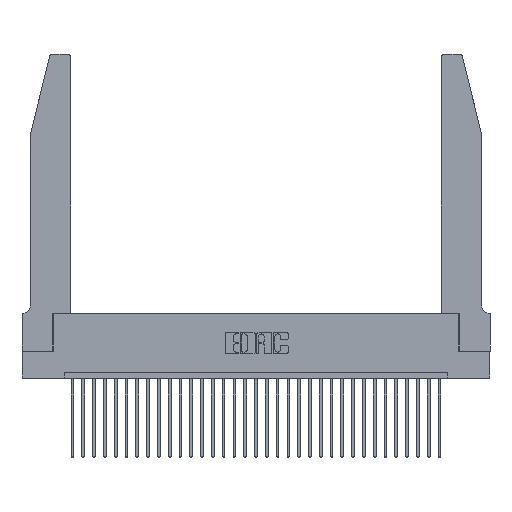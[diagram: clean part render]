
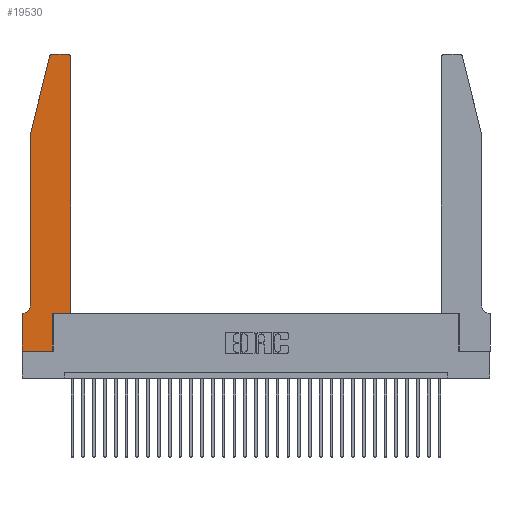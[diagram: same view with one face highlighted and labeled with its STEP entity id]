
A CAD part, top view. The second image highlights one B-rep face of the part: STEP entity #19530.
In plain terms, the highlighted planar face has unit normal (0, 0, 1).
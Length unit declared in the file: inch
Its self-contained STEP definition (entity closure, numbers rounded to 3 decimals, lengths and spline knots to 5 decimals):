
#37 = LINE ( 'NONE', #31479, #9733 ) ;
#382 = CARTESIAN_POINT ( 'NONE',  ( 0.0055, 0.35, 0.37 ) ) ;
#477 = ORIENTED_EDGE ( 'NONE', *, *, #24067, .T. ) ;
#713 = VERTEX_POINT ( 'NONE', #25484 ) ;
#748 = LINE ( 'NONE', #21684, #1137 ) ;
#1137 = VECTOR ( 'NONE', #14346, 39.37008 ) ;
#1479 = EDGE_LOOP ( 'NONE', ( #14843, #12441, #16678, #8493, #11657, #11386, #14791, #8676, #29667, #477, #28879, #24973 ) ) ;
#1513 = CARTESIAN_POINT ( 'NONE',  ( 0.284, 2.75, 0.37 ) ) ;
#1635 = CARTESIAN_POINT ( 'NONE',  ( 0.4505, 0.35, 0.37 ) ) ;
#1834 = AXIS2_PLACEMENT_3D ( 'NONE', #31867, #12397, #14784 ) ;
#1895 = VECTOR ( 'NONE', #10445, 39.37008 ) ;
#2207 = DIRECTION ( 'NONE',  ( 0., 1., 0. ) ) ;
#2646 = LINE ( 'NONE', #12282, #1895 ) ;
#2649 = CARTESIAN_POINT ( 'NONE',  ( 0.4505, 2.72, 0.37 ) ) ;
#2924 = DIRECTION ( 'NONE',  ( 0., 0., -1. ) ) ;
#3272 = VERTEX_POINT ( 'NONE', #19927 ) ;
#3446 = CARTESIAN_POINT ( 'NONE',  ( 0.0755, 0.42, 0.37 ) ) ;
#3865 = VERTEX_POINT ( 'NONE', #7511 ) ;
#4053 = CARTESIAN_POINT ( 'NONE',  ( 0.4505, 0.35, 0.37 ) ) ;
#4207 = DIRECTION ( 'NONE',  ( 0., 1., 0. ) ) ;
#4376 = EDGE_CURVE ( 'NONE', #12136, #10088, #5441, .T. ) ;
#4532 = DIRECTION ( 'NONE',  ( 1., 0., 0. ) ) ;
#4702 = CIRCLE ( 'NONE', #26055, 0.03 ) ;
#5030 = DIRECTION ( 'NONE',  ( -1., 0., 0. ) ) ;
#5145 = EDGE_CURVE ( 'NONE', #3272, #30229, #15882, .T. ) ;
#5441 = LINE ( 'NONE', #31015, #24458 ) ;
#7511 = CARTESIAN_POINT ( 'NONE',  ( 0., 0.35, 0.37 ) ) ;
#7933 = EDGE_CURVE ( 'NONE', #28340, #26289, #18375, .T. ) ;
#8493 = ORIENTED_EDGE ( 'NONE', *, *, #7933, .T. ) ;
#8676 = ORIENTED_EDGE ( 'NONE', *, *, #4376, .T. ) ;
#9013 = CARTESIAN_POINT ( 'NONE',  ( 0.2865, 0.35, 0.37 ) ) ;
#9733 = VECTOR ( 'NONE', #31569, 39.37008 ) ;
#10088 = VERTEX_POINT ( 'NONE', #22272 ) ;
#10445 = DIRECTION ( 'NONE',  ( -1., 0., 0. ) ) ;
#10763 = LINE ( 'NONE', #9013, #25900 ) ;
#11386 = ORIENTED_EDGE ( 'NONE', *, *, #17923, .T. ) ;
#11657 = ORIENTED_EDGE ( 'NONE', *, *, #12007, .T. ) ;
#11749 = CIRCLE ( 'NONE', #19691, 0.07 ) ;
#12007 = EDGE_CURVE ( 'NONE', #26289, #15824, #11749, .T. ) ;
#12136 = VERTEX_POINT ( 'NONE', #26726 ) ;
#12211 = VECTOR ( 'NONE', #29245, 39.37008 ) ;
#12282 = CARTESIAN_POINT ( 'NONE',  ( 0.0755, 0.35, 0.37 ) ) ;
#12397 = DIRECTION ( 'NONE',  ( 0., 0., 1. ) ) ;
#12441 = ORIENTED_EDGE ( 'NONE', *, *, #22831, .T. ) ;
#12475 = EDGE_CURVE ( 'NONE', #3865, #12136, #37, .T. ) ;
#13632 = DIRECTION ( 'NONE',  ( 0., 0., 1. ) ) ;
#14346 = DIRECTION ( 'NONE',  ( 1., 0., 0. ) ) ;
#14416 = DIRECTION ( 'NONE',  ( -1., 0., 0. ) ) ;
#14736 = VERTEX_POINT ( 'NONE', #2649 ) ;
#14784 = DIRECTION ( 'NONE',  ( 1., 0., 0. ) ) ;
#14791 = ORIENTED_EDGE ( 'NONE', *, *, #12475, .T. ) ;
#14843 = ORIENTED_EDGE ( 'NONE', *, *, #5145, .T. ) ;
#15542 = CARTESIAN_POINT ( 'NONE',  ( 0.0755, 2., 0.37 ) ) ;
#15824 = VERTEX_POINT ( 'NONE', #382 ) ;
#15882 = LINE ( 'NONE', #31395, #29079 ) ;
#15890 = DIRECTION ( 'NONE',  ( 1., 0., 0. ) ) ;
#16103 = DIRECTION ( 'NONE',  ( -0.239, -0.971, 0. ) ) ;
#16678 = ORIENTED_EDGE ( 'NONE', *, *, #22624, .T. ) ;
#16745 = VECTOR ( 'NONE', #16103, 39.37008 ) ;
#16967 = DIRECTION ( 'NONE',  ( 0., 0., 1. ) ) ;
#17652 = CARTESIAN_POINT ( 'NONE',  ( 0.0055, 0.42, 0.37 ) ) ;
#17923 = EDGE_CURVE ( 'NONE', #15824, #3865, #2646, .T. ) ;
#18356 = CARTESIAN_POINT ( 'NONE',  ( 0.0755, 2., 0.37 ) ) ;
#18375 = LINE ( 'NONE', #15542, #12211 ) ;
#18453 = VECTOR ( 'NONE', #2207, 39.37008 ) ;
#18917 = DIRECTION ( 'NONE',  ( 1., 0., 0. ) ) ;
#19530 = ADVANCED_FACE ( 'NONE', ( #32007 ), #29425, .T. ) ;
#19624 = LINE ( 'NONE', #4053, #18453 ) ;
#19691 = AXIS2_PLACEMENT_3D ( 'NONE', #17652, #2924, #5030 ) ;
#19927 = CARTESIAN_POINT ( 'NONE',  ( 0.4205, 2.75, 0.37 ) ) ;
#20639 = CARTESIAN_POINT ( 'NONE',  ( 0.0755, 2., 0.37 ) ) ;
#21078 = CARTESIAN_POINT ( 'NONE',  ( 0.4205, 2.72, 0.37 ) ) ;
#21405 = LINE ( 'NONE', #18356, #16745 ) ;
#21684 = CARTESIAN_POINT ( 'NONE',  ( 0.4505, 0.35, 0.37 ) ) ;
#22117 = VERTEX_POINT ( 'NONE', #1635 ) ;
#22272 = CARTESIAN_POINT ( 'NONE',  ( 0.2865, 0., 0.37 ) ) ;
#22624 = EDGE_CURVE ( 'NONE', #28176, #28340, #21405, .T. ) ;
#22831 = EDGE_CURVE ( 'NONE', #30229, #28176, #28735, .T. ) ;
#23986 = AXIS2_PLACEMENT_3D ( 'NONE', #29942, #16967, #4532 ) ;
#24067 = EDGE_CURVE ( 'NONE', #713, #22117, #748, .T. ) ;
#24458 = VECTOR ( 'NONE', #18917, 39.37008 ) ;
#24973 = ORIENTED_EDGE ( 'NONE', *, *, #28253, .T. ) ;
#25484 = CARTESIAN_POINT ( 'NONE',  ( 0.2865, 0.35, 0.37 ) ) ;
#25900 = VECTOR ( 'NONE', #4207, 39.37008 ) ;
#26055 = AXIS2_PLACEMENT_3D ( 'NONE', #21078, #13632, #15890 ) ;
#26289 = VERTEX_POINT ( 'NONE', #3446 ) ;
#26726 = CARTESIAN_POINT ( 'NONE',  ( 0., 0., 0.37 ) ) ;
#27673 = CARTESIAN_POINT ( 'NONE',  ( 0.25487, 2.72718, 0.37 ) ) ;
#28176 = VERTEX_POINT ( 'NONE', #27673 ) ;
#28253 = EDGE_CURVE ( 'NONE', #14736, #3272, #4702, .T. ) ;
#28340 = VERTEX_POINT ( 'NONE', #20639 ) ;
#28735 = CIRCLE ( 'NONE', #1834, 0.03 ) ;
#28879 = ORIENTED_EDGE ( 'NONE', *, *, #31034, .T. ) ;
#29079 = VECTOR ( 'NONE', #14416, 39.37008 ) ;
#29245 = DIRECTION ( 'NONE',  ( 0., -1., 0. ) ) ;
#29425 = PLANE ( 'NONE',  #23986 ) ;
#29667 = ORIENTED_EDGE ( 'NONE', *, *, #30302, .T. ) ;
#29942 = CARTESIAN_POINT ( 'NONE',  ( 0., 0.35, 0.37 ) ) ;
#30229 = VERTEX_POINT ( 'NONE', #1513 ) ;
#30302 = EDGE_CURVE ( 'NONE', #10088, #713, #10763, .T. ) ;
#31015 = CARTESIAN_POINT ( 'NONE',  ( 0., 0., 0.37 ) ) ;
#31034 = EDGE_CURVE ( 'NONE', #22117, #14736, #19624, .T. ) ;
#31395 = CARTESIAN_POINT ( 'NONE',  ( 0.2605, 2.75, 0.37 ) ) ;
#31479 = CARTESIAN_POINT ( 'NONE',  ( 0., 0., 0.37 ) ) ;
#31569 = DIRECTION ( 'NONE',  ( 0., -1., 0. ) ) ;
#31867 = CARTESIAN_POINT ( 'NONE',  ( 0.284, 2.72, 0.37 ) ) ;
#32007 = FACE_OUTER_BOUND ( 'NONE', #1479, .T. ) ;
